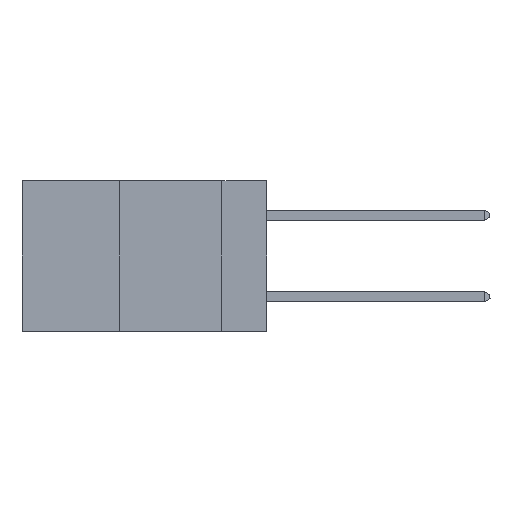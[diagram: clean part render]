
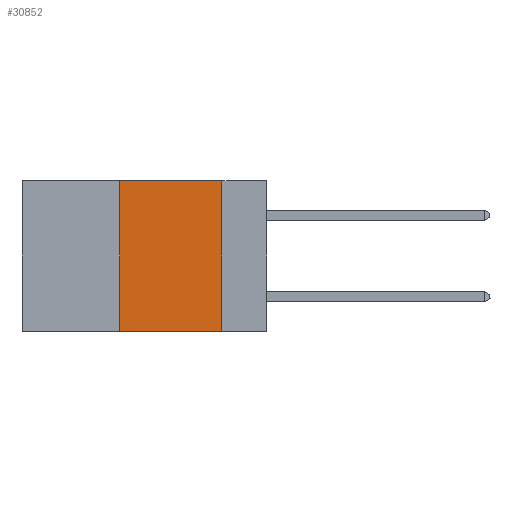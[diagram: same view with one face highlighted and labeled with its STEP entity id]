
A CAD part, left-side view. The second image highlights one B-rep face of the part: STEP entity #30852.
In plain terms, the highlighted planar face has unit normal (-1, 0, 0).
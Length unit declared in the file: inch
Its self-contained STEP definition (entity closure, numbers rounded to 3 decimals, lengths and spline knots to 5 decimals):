
#1044 = CARTESIAN_POINT ( 'NONE',  ( 0., 0.11, -0.37 ) ) ;
#1516 = CARTESIAN_POINT ( 'NONE',  ( 0., 0.11, 0. ) ) ;
#1917 = LINE ( 'NONE', #28118, #14852 ) ;
#3499 = PLANE ( 'NONE',  #35543 ) ;
#3683 = EDGE_CURVE ( 'NONE', #26868, #18762, #32350, .T. ) ;
#4566 = VECTOR ( 'NONE', #9893, 39.37008 ) ;
#6378 = DIRECTION ( 'NONE',  ( 0., 0., 1. ) ) ;
#7180 = LINE ( 'NONE', #15159, #4566 ) ;
#8709 = EDGE_CURVE ( 'NONE', #22095, #9941, #7180, .T. ) ;
#9123 = CARTESIAN_POINT ( 'NONE',  ( 0., 0.11, 0. ) ) ;
#9893 = DIRECTION ( 'NONE',  ( 0., -1., 0. ) ) ;
#9941 = VERTEX_POINT ( 'NONE', #9123 ) ;
#14852 = VECTOR ( 'NONE', #6378, 39.37008 ) ;
#15159 = CARTESIAN_POINT ( 'NONE',  ( 0., 0.6, 0. ) ) ;
#15932 = ORIENTED_EDGE ( 'NONE', *, *, #3683, .T. ) ;
#16813 = EDGE_CURVE ( 'NONE', #26868, #22095, #1917, .T. ) ;
#17262 = DIRECTION ( 'NONE',  ( 0., 0., -1. ) ) ;
#17757 = LINE ( 'NONE', #1516, #30306 ) ;
#18762 = VERTEX_POINT ( 'NONE', #1044 ) ;
#19144 = EDGE_LOOP ( 'NONE', ( #32322, #29501, #35596, #15932 ) ) ;
#19444 = CARTESIAN_POINT ( 'NONE',  ( 0., 0.6, -0.37 ) ) ;
#20138 = CARTESIAN_POINT ( 'NONE',  ( 0., 0.6, 0. ) ) ;
#22095 = VERTEX_POINT ( 'NONE', #29351 ) ;
#24904 = FACE_OUTER_BOUND ( 'NONE', #19144, .T. ) ;
#25000 = VECTOR ( 'NONE', #30895, 39.37008 ) ;
#26868 = VERTEX_POINT ( 'NONE', #33079 ) ;
#28118 = CARTESIAN_POINT ( 'NONE',  ( 0., 0.36, 0. ) ) ;
#29351 = CARTESIAN_POINT ( 'NONE',  ( 0., 0.36, 0. ) ) ;
#29501 = ORIENTED_EDGE ( 'NONE', *, *, #8709, .F. ) ;
#30306 = VECTOR ( 'NONE', #34910, 39.37008 ) ;
#30852 = ADVANCED_FACE ( 'NONE', ( #24904 ), #3499, .F. ) ;
#30895 = DIRECTION ( 'NONE',  ( 0., -1., 0. ) ) ;
#31115 = DIRECTION ( 'NONE',  ( 1., 0., 0. ) ) ;
#32322 = ORIENTED_EDGE ( 'NONE', *, *, #32670, .F. ) ;
#32350 = LINE ( 'NONE', #19444, #25000 ) ;
#32670 = EDGE_CURVE ( 'NONE', #9941, #18762, #17757, .T. ) ;
#33079 = CARTESIAN_POINT ( 'NONE',  ( 0., 0.36, -0.37 ) ) ;
#34910 = DIRECTION ( 'NONE',  ( 0., 0., -1. ) ) ;
#35543 = AXIS2_PLACEMENT_3D ( 'NONE', #20138, #31115, #17262 ) ;
#35596 = ORIENTED_EDGE ( 'NONE', *, *, #16813, .F. ) ;
